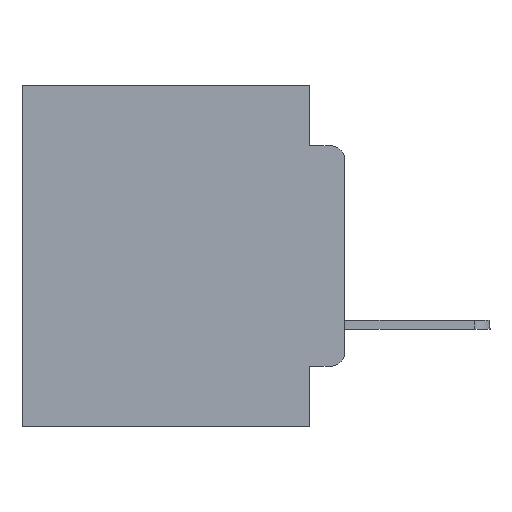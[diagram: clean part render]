
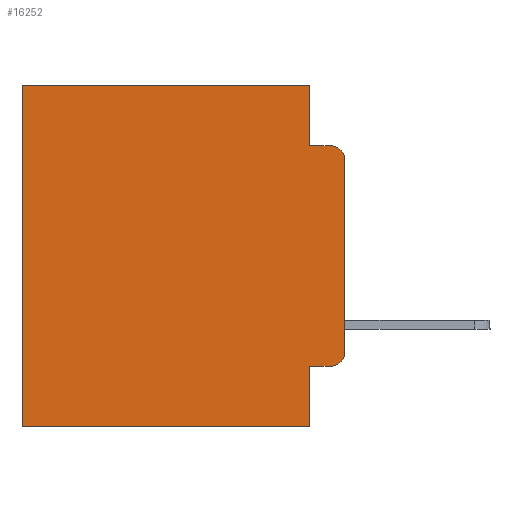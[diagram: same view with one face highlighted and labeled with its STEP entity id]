
A CAD part, left-side view. The second image highlights one B-rep face of the part: STEP entity #16252.
In plain terms, the highlighted planar face has unit normal (-1, 0, 0).
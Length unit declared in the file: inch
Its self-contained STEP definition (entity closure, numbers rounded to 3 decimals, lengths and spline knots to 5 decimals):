
#540 = ORIENTED_EDGE ( 'NONE', *, *, #10657, .F. ) ;
#1081 = VERTEX_POINT ( 'NONE', #19881 ) ;
#1446 = EDGE_CURVE ( 'NONE', #14287, #28473, #6841, .T. ) ;
#1788 = CARTESIAN_POINT ( 'NONE',  ( 0.298, 0., 0. ) ) ;
#2242 = CARTESIAN_POINT ( 'NONE',  ( 0.298, 0.051, 0. ) ) ;
#3341 = VERTEX_POINT ( 'NONE', #24246 ) ;
#3496 = VECTOR ( 'NONE', #17453, 39.37008 ) ;
#3587 = EDGE_CURVE ( 'NONE', #1081, #3341, #28302, .T. ) ;
#4488 = CIRCLE ( 'NONE', #7779, 0.02 ) ;
#4884 = LINE ( 'NONE', #18410, #18987 ) ;
#5152 = VECTOR ( 'NONE', #8084, 39.37008 ) ;
#5253 = CARTESIAN_POINT ( 'NONE',  ( 0.298, 0.02, -0.0885 ) ) ;
#5297 = ORIENTED_EDGE ( 'NONE', *, *, #27744, .T. ) ;
#5699 = CARTESIAN_POINT ( 'NONE',  ( 0.298, 0.051, 0. ) ) ;
#5713 = DIRECTION ( 'NONE',  ( 0., -1., 0. ) ) ;
#6841 = CIRCLE ( 'NONE', #9184, 0.02 ) ;
#7037 = EDGE_CURVE ( 'NONE', #15008, #23994, #16459, .T. ) ;
#7378 = DIRECTION ( 'NONE',  ( 0., 0., -1. ) ) ;
#7779 = AXIS2_PLACEMENT_3D ( 'NONE', #17566, #8886, #9021 ) ;
#7780 = ORIENTED_EDGE ( 'NONE', *, *, #24145, .F. ) ;
#8035 = DIRECTION ( 'NONE',  ( 0., 0., -1. ) ) ;
#8084 = DIRECTION ( 'NONE',  ( 0., 1., 0. ) ) ;
#8645 = VECTOR ( 'NONE', #17932, 39.37008 ) ;
#8886 = DIRECTION ( 'NONE',  ( -1., 0., 0. ) ) ;
#9021 = DIRECTION ( 'NONE',  ( 0., 0., -1. ) ) ;
#9184 = AXIS2_PLACEMENT_3D ( 'NONE', #21450, #19525, #8035 ) ;
#9215 = EDGE_CURVE ( 'NONE', #18723, #28473, #18084, .T. ) ;
#9481 = ORIENTED_EDGE ( 'NONE', *, *, #1446, .T. ) ;
#10436 = CARTESIAN_POINT ( 'NONE',  ( 0.298, 0.051, -0.4115 ) ) ;
#10583 = VERTEX_POINT ( 'NONE', #2242 ) ;
#10657 = EDGE_CURVE ( 'NONE', #15008, #20868, #4884, .T. ) ;
#10690 = LINE ( 'NONE', #5699, #3496 ) ;
#11498 = PLANE ( 'NONE',  #11816 ) ;
#11816 = AXIS2_PLACEMENT_3D ( 'NONE', #25052, #23287, #7378 ) ;
#11934 = FACE_OUTER_BOUND ( 'NONE', #12345, .T. ) ;
#12054 = VECTOR ( 'NONE', #17790, 39.37008 ) ;
#12109 = ORIENTED_EDGE ( 'NONE', *, *, #13690, .F. ) ;
#12256 = CARTESIAN_POINT ( 'NONE',  ( 0.298, 0.473, 0. ) ) ;
#12345 = EDGE_LOOP ( 'NONE', ( #7780, #9481, #25687, #21995, #19451, #13752, #12109, #540, #16177, #5297 ) ) ;
#13200 = VECTOR ( 'NONE', #5713, 39.37008 ) ;
#13690 = EDGE_CURVE ( 'NONE', #20868, #3341, #26047, .T. ) ;
#13752 = ORIENTED_EDGE ( 'NONE', *, *, #3587, .T. ) ;
#14287 = VERTEX_POINT ( 'NONE', #27206 ) ;
#14608 = EDGE_CURVE ( 'NONE', #10583, #1081, #22261, .T. ) ;
#15008 = VERTEX_POINT ( 'NONE', #10436 ) ;
#15413 = CARTESIAN_POINT ( 'NONE',  ( 0.298, 0., 0. ) ) ;
#15706 = LINE ( 'NONE', #15413, #12054 ) ;
#15750 = DIRECTION ( 'NONE',  ( 0., 0., -1. ) ) ;
#16177 = ORIENTED_EDGE ( 'NONE', *, *, #7037, .T. ) ;
#16252 = ADVANCED_FACE ( 'NONE', ( #11934 ), #11498, .F. ) ;
#16459 = LINE ( 'NONE', #25460, #13200 ) ;
#17453 = DIRECTION ( 'NONE',  ( 0., 0., -1. ) ) ;
#17530 = DIRECTION ( 'NONE',  ( 0., 1., 0. ) ) ;
#17566 = CARTESIAN_POINT ( 'NONE',  ( 0.298, 0.02, -0.3915 ) ) ;
#17790 = DIRECTION ( 'NONE',  ( 0., 0., -1. ) ) ;
#17932 = DIRECTION ( 'NONE',  ( 0., -1., 0. ) ) ;
#18084 = LINE ( 'NONE', #19712, #8645 ) ;
#18410 = CARTESIAN_POINT ( 'NONE',  ( 0.298, 0.051, 0. ) ) ;
#18723 = VERTEX_POINT ( 'NONE', #21708 ) ;
#18987 = VECTOR ( 'NONE', #15750, 39.37008 ) ;
#19451 = ORIENTED_EDGE ( 'NONE', *, *, #14608, .T. ) ;
#19525 = DIRECTION ( 'NONE',  ( -1., 0., 0. ) ) ;
#19620 = CARTESIAN_POINT ( 'NONE',  ( 0.298, 0.02, -0.4115 ) ) ;
#19712 = CARTESIAN_POINT ( 'NONE',  ( 0.298, 0.051, -0.0885 ) ) ;
#19881 = CARTESIAN_POINT ( 'NONE',  ( 0.298, 0.473, 0. ) ) ;
#20868 = VERTEX_POINT ( 'NONE', #25408 ) ;
#21450 = CARTESIAN_POINT ( 'NONE',  ( 0.298, 0.02, -0.1085 ) ) ;
#21708 = CARTESIAN_POINT ( 'NONE',  ( 0.298, 0.051, -0.0885 ) ) ;
#21929 = CARTESIAN_POINT ( 'NONE',  ( 0.298, 0., -0.5 ) ) ;
#21995 = ORIENTED_EDGE ( 'NONE', *, *, #27187, .F. ) ;
#22261 = LINE ( 'NONE', #1788, #23999 ) ;
#23287 = DIRECTION ( 'NONE',  ( 1., 0., 0. ) ) ;
#23994 = VERTEX_POINT ( 'NONE', #19620 ) ;
#23999 = VECTOR ( 'NONE', #17530, 39.37008 ) ;
#24145 = EDGE_CURVE ( 'NONE', #14287, #24773, #15706, .T. ) ;
#24246 = CARTESIAN_POINT ( 'NONE',  ( 0.298, 0.473, -0.5 ) ) ;
#24524 = CARTESIAN_POINT ( 'NONE',  ( 0.298, 0., -0.3915 ) ) ;
#24773 = VERTEX_POINT ( 'NONE', #24524 ) ;
#25052 = CARTESIAN_POINT ( 'NONE',  ( 0.298, 0., 0. ) ) ;
#25408 = CARTESIAN_POINT ( 'NONE',  ( 0.298, 0.051, -0.5 ) ) ;
#25460 = CARTESIAN_POINT ( 'NONE',  ( 0.298, 0.051, -0.4115 ) ) ;
#25687 = ORIENTED_EDGE ( 'NONE', *, *, #9215, .F. ) ;
#26047 = LINE ( 'NONE', #21929, #5152 ) ;
#26083 = DIRECTION ( 'NONE',  ( 0., 0., -1. ) ) ;
#27187 = EDGE_CURVE ( 'NONE', #10583, #18723, #10690, .T. ) ;
#27206 = CARTESIAN_POINT ( 'NONE',  ( 0.298, 0., -0.1085 ) ) ;
#27744 = EDGE_CURVE ( 'NONE', #23994, #24773, #4488, .T. ) ;
#28302 = LINE ( 'NONE', #12256, #28597 ) ;
#28473 = VERTEX_POINT ( 'NONE', #5253 ) ;
#28597 = VECTOR ( 'NONE', #26083, 39.37008 ) ;
